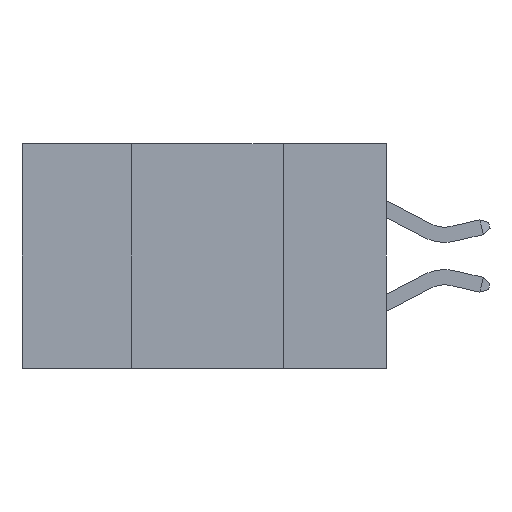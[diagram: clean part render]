
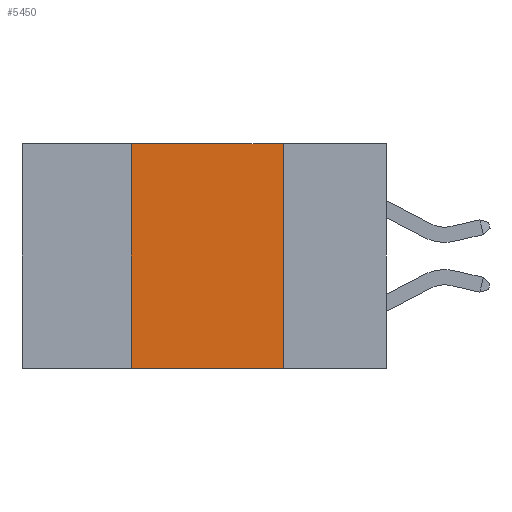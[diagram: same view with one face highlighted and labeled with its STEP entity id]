
A CAD part, left-side view. The second image highlights one B-rep face of the part: STEP entity #5450.
In plain terms, the highlighted planar face has unit normal (-1, 0, 0).
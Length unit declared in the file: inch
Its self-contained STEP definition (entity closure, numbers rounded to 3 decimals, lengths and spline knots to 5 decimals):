
#37 = CARTESIAN_POINT ( 'NONE',  ( 0., 0.6, 0. ) ) ;
#611 = DIRECTION ( 'NONE',  ( 0., 0., 1. ) ) ;
#1905 = PLANE ( 'NONE',  #4321 ) ;
#2004 = DIRECTION ( 'NONE',  ( 0., -1., 0. ) ) ;
#2128 = CARTESIAN_POINT ( 'NONE',  ( 0., 0.42, -0.37 ) ) ;
#2154 = VECTOR ( 'NONE', #7566, 39.37008 ) ;
#2188 = CARTESIAN_POINT ( 'NONE',  ( 0., 0.42, 0. ) ) ;
#2578 = VERTEX_POINT ( 'NONE', #2128 ) ;
#2733 = LINE ( 'NONE', #2782, #3452 ) ;
#2782 = CARTESIAN_POINT ( 'NONE',  ( 0., 0.17, -0.37 ) ) ;
#2963 = EDGE_LOOP ( 'NONE', ( #6439, #8079, #8744, #8217 ) ) ;
#3452 = VECTOR ( 'NONE', #7446, 39.37008 ) ;
#3749 = VECTOR ( 'NONE', #2004, 39.37008 ) ;
#3770 = LINE ( 'NONE', #6776, #2154 ) ;
#4321 = AXIS2_PLACEMENT_3D ( 'NONE', #7218, #8031, #8893 ) ;
#4681 = VERTEX_POINT ( 'NONE', #9064 ) ;
#5450 = ADVANCED_FACE ( 'NONE', ( #8740 ), #1905, .F. ) ;
#6199 = EDGE_CURVE ( 'NONE', #4681, #9141, #2733, .T. ) ;
#6439 = ORIENTED_EDGE ( 'NONE', *, *, #6199, .F. ) ;
#6447 = EDGE_CURVE ( 'NONE', #2578, #9523, #8247, .T. ) ;
#6776 = CARTESIAN_POINT ( 'NONE',  ( 0., 0.6, -0.37 ) ) ;
#6929 = LINE ( 'NONE', #37, #3749 ) ;
#7092 = EDGE_CURVE ( 'NONE', #9523, #4681, #6929, .T. ) ;
#7218 = CARTESIAN_POINT ( 'NONE',  ( 0., 0.6, 0. ) ) ;
#7267 = EDGE_CURVE ( 'NONE', #2578, #9141, #3770, .T. ) ;
#7446 = DIRECTION ( 'NONE',  ( 0., 0., -1. ) ) ;
#7494 = CARTESIAN_POINT ( 'NONE',  ( 0., 0.42, -0.37 ) ) ;
#7566 = DIRECTION ( 'NONE',  ( 0., -1., 0. ) ) ;
#8018 = VECTOR ( 'NONE', #611, 39.37008 ) ;
#8031 = DIRECTION ( 'NONE',  ( 1., 0., 0. ) ) ;
#8079 = ORIENTED_EDGE ( 'NONE', *, *, #7092, .F. ) ;
#8217 = ORIENTED_EDGE ( 'NONE', *, *, #7267, .T. ) ;
#8247 = LINE ( 'NONE', #7494, #8018 ) ;
#8740 = FACE_OUTER_BOUND ( 'NONE', #2963, .T. ) ;
#8744 = ORIENTED_EDGE ( 'NONE', *, *, #6447, .F. ) ;
#8893 = DIRECTION ( 'NONE',  ( 0., 0., -1. ) ) ;
#9064 = CARTESIAN_POINT ( 'NONE',  ( 0., 0.17, 0. ) ) ;
#9141 = VERTEX_POINT ( 'NONE', #9218 ) ;
#9218 = CARTESIAN_POINT ( 'NONE',  ( 0., 0.17, -0.37 ) ) ;
#9523 = VERTEX_POINT ( 'NONE', #2188 ) ;
